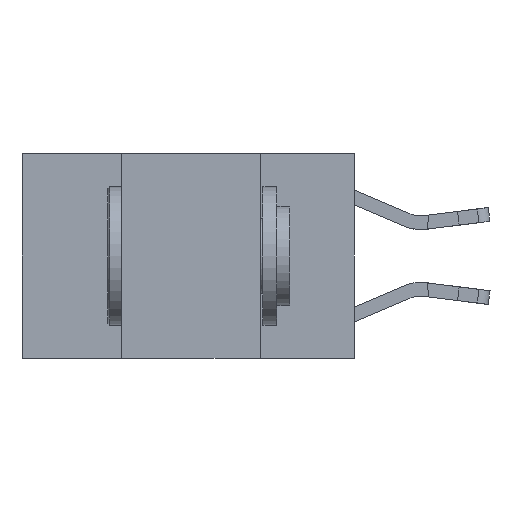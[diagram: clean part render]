
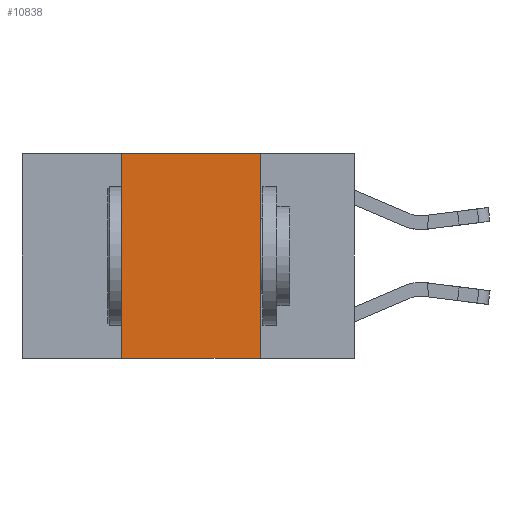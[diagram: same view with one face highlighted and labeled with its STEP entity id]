
A CAD part, left-side view. The second image highlights one B-rep face of the part: STEP entity #10838.
In plain terms, the highlighted planar face has unit normal (-1, 0, 0).
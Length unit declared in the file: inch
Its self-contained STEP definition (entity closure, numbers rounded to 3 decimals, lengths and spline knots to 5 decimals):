
#638 = DIRECTION ( 'NONE',  ( 0., 0., -1. ) ) ;
#850 = EDGE_LOOP ( 'NONE', ( #10491, #8781, #11152, #13478 ) ) ;
#1344 = CARTESIAN_POINT ( 'NONE',  ( 0., 0.42, 0. ) ) ;
#1888 = CARTESIAN_POINT ( 'NONE',  ( 0., 0.6, -0.37 ) ) ;
#2077 = VECTOR ( 'NONE', #2829, 39.37008 ) ;
#2369 = EDGE_CURVE ( 'NONE', #6973, #3789, #16946, .T. ) ;
#2707 = CARTESIAN_POINT ( 'NONE',  ( 0., 0.42, -0.37 ) ) ;
#2829 = DIRECTION ( 'NONE',  ( 0., 0., 1. ) ) ;
#2847 = CARTESIAN_POINT ( 'NONE',  ( 0., 0.17, -0.37 ) ) ;
#3104 = VERTEX_POINT ( 'NONE', #16737 ) ;
#3789 = VERTEX_POINT ( 'NONE', #2847 ) ;
#4753 = CARTESIAN_POINT ( 'NONE',  ( 0., 0.6, 0. ) ) ;
#5263 = PLANE ( 'NONE',  #12288 ) ;
#5754 = LINE ( 'NONE', #4753, #10369 ) ;
#6677 = DIRECTION ( 'NONE',  ( 1., 0., 0. ) ) ;
#6973 = VERTEX_POINT ( 'NONE', #13258 ) ;
#8657 = EDGE_CURVE ( 'NONE', #17438, #3104, #10043, .T. ) ;
#8781 = ORIENTED_EDGE ( 'NONE', *, *, #14817, .F. ) ;
#9596 = VECTOR ( 'NONE', #638, 39.37008 ) ;
#10043 = LINE ( 'NONE', #1344, #2077 ) ;
#10369 = VECTOR ( 'NONE', #11757, 39.37008 ) ;
#10371 = DIRECTION ( 'NONE',  ( 0., -1., 0. ) ) ;
#10491 = ORIENTED_EDGE ( 'NONE', *, *, #2369, .F. ) ;
#10600 = CARTESIAN_POINT ( 'NONE',  ( 0., 0.17, 0. ) ) ;
#10838 = ADVANCED_FACE ( 'NONE', ( #10845 ), #5263, .F. ) ;
#10845 = FACE_OUTER_BOUND ( 'NONE', #850, .T. ) ;
#11152 = ORIENTED_EDGE ( 'NONE', *, *, #8657, .F. ) ;
#11757 = DIRECTION ( 'NONE',  ( 0., -1., 0. ) ) ;
#12288 = AXIS2_PLACEMENT_3D ( 'NONE', #15047, #6677, #16419 ) ;
#12817 = EDGE_CURVE ( 'NONE', #17438, #3789, #17015, .T. ) ;
#13258 = CARTESIAN_POINT ( 'NONE',  ( 0., 0.17, 0. ) ) ;
#13373 = VECTOR ( 'NONE', #10371, 39.37008 ) ;
#13478 = ORIENTED_EDGE ( 'NONE', *, *, #12817, .T. ) ;
#14817 = EDGE_CURVE ( 'NONE', #3104, #6973, #5754, .T. ) ;
#15047 = CARTESIAN_POINT ( 'NONE',  ( 0., 0.6, 0. ) ) ;
#16419 = DIRECTION ( 'NONE',  ( 0., 0., -1. ) ) ;
#16737 = CARTESIAN_POINT ( 'NONE',  ( 0., 0.42, 0. ) ) ;
#16946 = LINE ( 'NONE', #10600, #9596 ) ;
#17015 = LINE ( 'NONE', #1888, #13373 ) ;
#17438 = VERTEX_POINT ( 'NONE', #2707 ) ;
